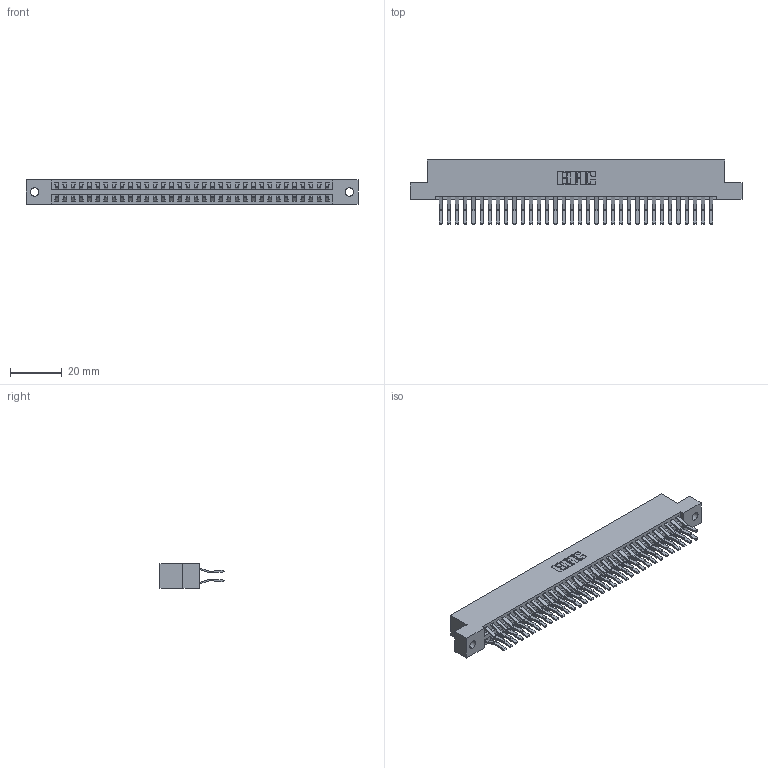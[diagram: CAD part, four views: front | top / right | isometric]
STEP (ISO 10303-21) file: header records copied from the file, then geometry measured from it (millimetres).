
FILE_DESCRIPTION (( 'STEP AP203' ), '1' );
FILE_NAME ('346-068-560-202.STEP', '2022-05-24T20:21:00', ( '' ), ( '' ), 'SwSTEP 2.0', 'SolidWorks 2020', '' );
FILE_SCHEMA (( 'CONFIG_CONTROL_DESIGN' ));
Length unit declared in the file: inch
Products named in the file (3): 346 Part_Flush Mounting Lugs - 0.128 Dia; 345-292-001_560 Tail; 346-068-560-202
Assembly tree (69 placements, depth 2):
  346-068-560-202
    346 Part_Flush Mounting Lugs - 0.128 Dia
    345-292-001_560 Tail  x68
Bounding box: 128.52 x 24.78 x 9.4 mm (x, y, z)
Volume: 12879.6 mm3; surface area: 18498 mm2
Topology: 69 solids, 69 shells, 3794 faces, 11277 edges, 7426 vertices
Faces by surface type: plane 2456, cylinder 1338
Entity records: 23357 total; most frequent: CARTESIAN_POINT 3860, ORIENTED_EDGE 3794, DIRECTION 3457, EDGE_CURVE 1897, LINE 1625, VECTOR 1625, VERTEX_POINT 1262, AXIS2_PLACEMENT_3D 916
